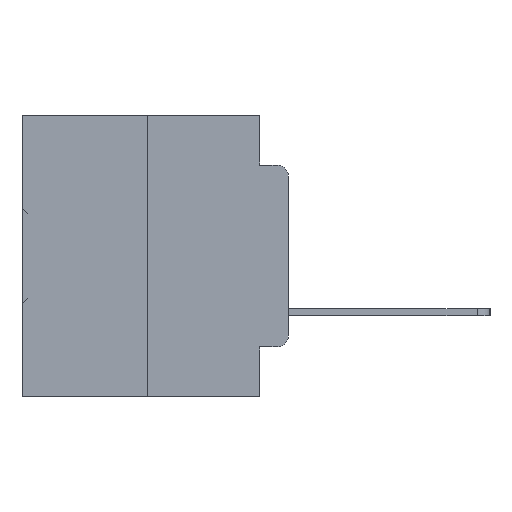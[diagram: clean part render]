
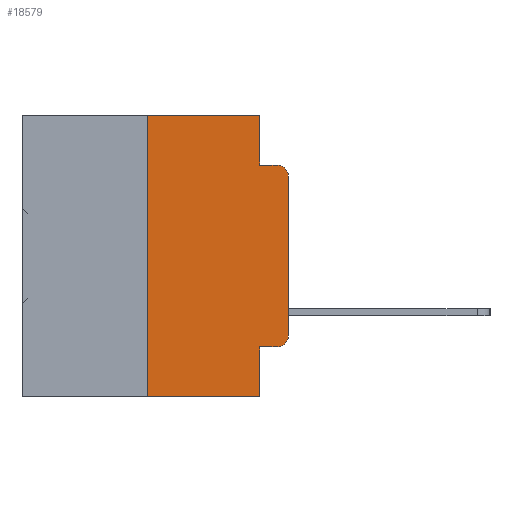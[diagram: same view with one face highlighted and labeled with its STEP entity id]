
A CAD part, left-side view. The second image highlights one B-rep face of the part: STEP entity #18579.
In plain terms, the highlighted planar face has unit normal (-1, 0, 0).
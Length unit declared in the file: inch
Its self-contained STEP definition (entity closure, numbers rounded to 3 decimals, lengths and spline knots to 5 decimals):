
#350 = EDGE_CURVE ( 'NONE', #16275, #18851, #30880, .T. ) ;
#1305 = EDGE_CURVE ( 'NONE', #11316, #14653, #35016, .T. ) ;
#1745 = CARTESIAN_POINT ( 'NONE',  ( 0., 0.051, -0.0885 ) ) ;
#1859 = CARTESIAN_POINT ( 'NONE',  ( 0., 0.25, 0. ) ) ;
#2137 = LINE ( 'NONE', #12452, #16000 ) ;
#3109 = CARTESIAN_POINT ( 'NONE',  ( 0., 0.051, -0.0885 ) ) ;
#3844 = VECTOR ( 'NONE', #26648, 39.37008 ) ;
#4018 = VERTEX_POINT ( 'NONE', #7139 ) ;
#5383 = ORIENTED_EDGE ( 'NONE', *, *, #31059, .T. ) ;
#5435 = PLANE ( 'NONE',  #22411 ) ;
#6675 = ORIENTED_EDGE ( 'NONE', *, *, #350, .F. ) ;
#7118 = ORIENTED_EDGE ( 'NONE', *, *, #29012, .T. ) ;
#7139 = CARTESIAN_POINT ( 'NONE',  ( 0., 0.051, 0. ) ) ;
#7166 = VERTEX_POINT ( 'NONE', #17630 ) ;
#7240 = CIRCLE ( 'NONE', #7789, 0.02 ) ;
#7789 = AXIS2_PLACEMENT_3D ( 'NONE', #9165, #28317, #11929 ) ;
#8728 = DIRECTION ( 'NONE',  ( 0., -1., 0. ) ) ;
#9095 = VECTOR ( 'NONE', #32295, 39.37008 ) ;
#9165 = CARTESIAN_POINT ( 'NONE',  ( 0., 0.02, -0.1085 ) ) ;
#9303 = ORIENTED_EDGE ( 'NONE', *, *, #35191, .F. ) ;
#9327 = DIRECTION ( 'NONE',  ( 0., 0., 1. ) ) ;
#9434 = CARTESIAN_POINT ( 'NONE',  ( 0., 0.02, -0.0885 ) ) ;
#10449 = VECTOR ( 'NONE', #8728, 39.37008 ) ;
#10817 = CARTESIAN_POINT ( 'NONE',  ( 0., 0.02, -0.3915 ) ) ;
#11316 = VERTEX_POINT ( 'NONE', #31150 ) ;
#11738 = LINE ( 'NONE', #25631, #25427 ) ;
#11929 = DIRECTION ( 'NONE',  ( 0., 0., -1. ) ) ;
#12257 = CARTESIAN_POINT ( 'NONE',  ( 0., 0.25, -0.5 ) ) ;
#12452 = CARTESIAN_POINT ( 'NONE',  ( 0., 0.051, 0. ) ) ;
#12537 = DIRECTION ( 'NONE',  ( 0., 0., -1. ) ) ;
#12655 = EDGE_CURVE ( 'NONE', #20098, #7166, #31337, .T. ) ;
#12726 = CARTESIAN_POINT ( 'NONE',  ( 0., 0., 0. ) ) ;
#13494 = EDGE_CURVE ( 'NONE', #20098, #21500, #32933, .T. ) ;
#13597 = DIRECTION ( 'NONE',  ( 0., 0., -1. ) ) ;
#14648 = EDGE_CURVE ( 'NONE', #4018, #16275, #2137, .T. ) ;
#14653 = VERTEX_POINT ( 'NONE', #15222 ) ;
#15222 = CARTESIAN_POINT ( 'NONE',  ( 0., 0., -0.1085 ) ) ;
#15776 = ORIENTED_EDGE ( 'NONE', *, *, #14648, .F. ) ;
#16000 = VECTOR ( 'NONE', #31483, 39.37008 ) ;
#16275 = VERTEX_POINT ( 'NONE', #3109 ) ;
#16561 = DIRECTION ( 'NONE',  ( 1., 0., 0. ) ) ;
#17630 = CARTESIAN_POINT ( 'NONE',  ( 0., 0.051, -0.5 ) ) ;
#17886 = ORIENTED_EDGE ( 'NONE', *, *, #1305, .T. ) ;
#18040 = EDGE_CURVE ( 'NONE', #26772, #7166, #33161, .T. ) ;
#18579 = ADVANCED_FACE ( 'NONE', ( #29807 ), #5435, .F. ) ;
#18763 = VECTOR ( 'NONE', #27327, 39.37008 ) ;
#18851 = VERTEX_POINT ( 'NONE', #9434 ) ;
#19092 = CARTESIAN_POINT ( 'NONE',  ( 0., 0.051, 0. ) ) ;
#20098 = VERTEX_POINT ( 'NONE', #12257 ) ;
#20318 = LINE ( 'NONE', #34150, #33841 ) ;
#20456 = ORIENTED_EDGE ( 'NONE', *, *, #23002, .T. ) ;
#20672 = VECTOR ( 'NONE', #9327, 39.37008 ) ;
#21500 = VERTEX_POINT ( 'NONE', #29862 ) ;
#22411 = AXIS2_PLACEMENT_3D ( 'NONE', #30128, #16561, #12537 ) ;
#22578 = CARTESIAN_POINT ( 'NONE',  ( 0., 0.051, -0.4115 ) ) ;
#22656 = VERTEX_POINT ( 'NONE', #27320 ) ;
#23002 = EDGE_CURVE ( 'NONE', #14653, #18851, #7240, .T. ) ;
#23892 = ORIENTED_EDGE ( 'NONE', *, *, #13494, .F. ) ;
#25127 = CARTESIAN_POINT ( 'NONE',  ( 0., 0.473, -0.5 ) ) ;
#25427 = VECTOR ( 'NONE', #31066, 39.37008 ) ;
#25631 = CARTESIAN_POINT ( 'NONE',  ( 0., 0.051, -0.4115 ) ) ;
#26453 = ORIENTED_EDGE ( 'NONE', *, *, #18040, .F. ) ;
#26648 = DIRECTION ( 'NONE',  ( 0., 0., 1. ) ) ;
#26772 = VERTEX_POINT ( 'NONE', #22578 ) ;
#27320 = CARTESIAN_POINT ( 'NONE',  ( 0., 0.02, -0.4115 ) ) ;
#27327 = DIRECTION ( 'NONE',  ( 0., 0., -1. ) ) ;
#28317 = DIRECTION ( 'NONE',  ( -1., 0., 0. ) ) ;
#29012 = EDGE_CURVE ( 'NONE', #22656, #11316, #31551, .T. ) ;
#29501 = AXIS2_PLACEMENT_3D ( 'NONE', #10817, #29916, #13597 ) ;
#29807 = FACE_OUTER_BOUND ( 'NONE', #31062, .T. ) ;
#29862 = CARTESIAN_POINT ( 'NONE',  ( 0., 0.25, 0. ) ) ;
#29916 = DIRECTION ( 'NONE',  ( -1., 0., 0. ) ) ;
#30128 = CARTESIAN_POINT ( 'NONE',  ( 0., 0.473, 0. ) ) ;
#30880 = LINE ( 'NONE', #1745, #9095 ) ;
#31059 = EDGE_CURVE ( 'NONE', #26772, #22656, #11738, .T. ) ;
#31062 = EDGE_LOOP ( 'NONE', ( #17886, #20456, #6675, #15776, #9303, #23892, #32739, #26453, #5383, #7118 ) ) ;
#31066 = DIRECTION ( 'NONE',  ( 0., -1., 0. ) ) ;
#31150 = CARTESIAN_POINT ( 'NONE',  ( 0., 0., -0.3915 ) ) ;
#31337 = LINE ( 'NONE', #25127, #10449 ) ;
#31483 = DIRECTION ( 'NONE',  ( 0., 0., -1. ) ) ;
#31551 = CIRCLE ( 'NONE', #29501, 0.02 ) ;
#31592 = DIRECTION ( 'NONE',  ( 0., -1., 0. ) ) ;
#32295 = DIRECTION ( 'NONE',  ( 0., -1., 0. ) ) ;
#32739 = ORIENTED_EDGE ( 'NONE', *, *, #12655, .T. ) ;
#32933 = LINE ( 'NONE', #1859, #3844 ) ;
#33161 = LINE ( 'NONE', #19092, #18763 ) ;
#33841 = VECTOR ( 'NONE', #31592, 39.37008 ) ;
#34150 = CARTESIAN_POINT ( 'NONE',  ( 0., 0.473, 0. ) ) ;
#35016 = LINE ( 'NONE', #12726, #20672 ) ;
#35191 = EDGE_CURVE ( 'NONE', #21500, #4018, #20318, .T. ) ;
